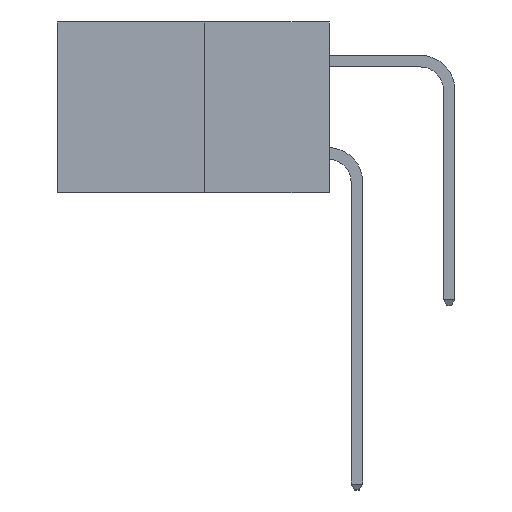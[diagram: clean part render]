
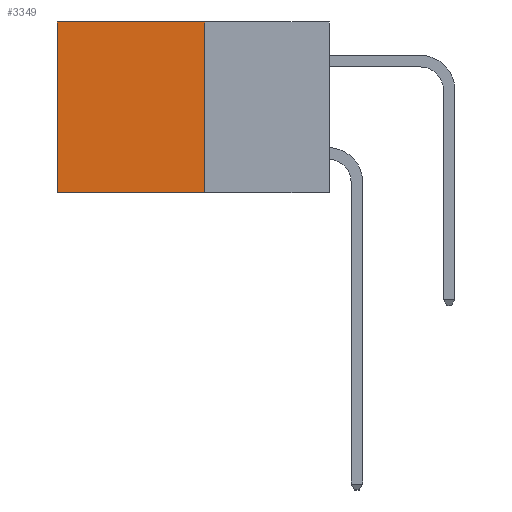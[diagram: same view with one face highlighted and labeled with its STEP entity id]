
A CAD part, left-side view. The second image highlights one B-rep face of the part: STEP entity #3349.
In plain terms, the highlighted planar face has unit normal (-1, 0, 0).
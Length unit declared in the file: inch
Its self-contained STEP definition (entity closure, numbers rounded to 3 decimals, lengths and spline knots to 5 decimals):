
#396 = LINE ( 'NONE', #4796, #4317 ) ;
#1114 = ORIENTED_EDGE ( 'NONE', *, *, #7311, .F. ) ;
#1299 = CARTESIAN_POINT ( 'NONE',  ( 0.277, 0.27, -0.37 ) ) ;
#1785 = LINE ( 'NONE', #10748, #14183 ) ;
#3349 = ADVANCED_FACE ( 'NONE', ( #7899 ), #6500, .F. ) ;
#3978 = DIRECTION ( 'NONE',  ( 0., 0., -1. ) ) ;
#4066 = ORIENTED_EDGE ( 'NONE', *, *, #15987, .F. ) ;
#4118 = AXIS2_PLACEMENT_3D ( 'NONE', #1299, #9331, #3978 ) ;
#4317 = VECTOR ( 'NONE', #13659, 39.37008 ) ;
#4387 = ORIENTED_EDGE ( 'NONE', *, *, #11610, .T. ) ;
#4666 = CARTESIAN_POINT ( 'NONE',  ( 0.277, 0.27, -0.37 ) ) ;
#4796 = CARTESIAN_POINT ( 'NONE',  ( 0.277, 0.27, 0. ) ) ;
#4923 = CARTESIAN_POINT ( 'NONE',  ( 0.277, 0.59, 0. ) ) ;
#5635 = EDGE_LOOP ( 'NONE', ( #4387, #4066, #1114, #10881 ) ) ;
#6076 = VERTEX_POINT ( 'NONE', #4923 ) ;
#6500 = PLANE ( 'NONE',  #4118 ) ;
#6636 = EDGE_CURVE ( 'NONE', #11282, #6076, #396, .T. ) ;
#7311 = EDGE_CURVE ( 'NONE', #11282, #11649, #13811, .T. ) ;
#7348 = LINE ( 'NONE', #8832, #13654 ) ;
#7899 = FACE_OUTER_BOUND ( 'NONE', #5635, .T. ) ;
#8777 = CARTESIAN_POINT ( 'NONE',  ( 0.277, 0.59, -0.37 ) ) ;
#8832 = CARTESIAN_POINT ( 'NONE',  ( 0.277, 0.27, -0.37 ) ) ;
#9331 = DIRECTION ( 'NONE',  ( 1., 0., 0. ) ) ;
#10033 = CARTESIAN_POINT ( 'NONE',  ( 0.277, 0.27, 0. ) ) ;
#10103 = DIRECTION ( 'NONE',  ( 0., 1., 0. ) ) ;
#10471 = VECTOR ( 'NONE', #12311, 39.37008 ) ;
#10748 = CARTESIAN_POINT ( 'NONE',  ( 0.277, 0.59, -0.37 ) ) ;
#10881 = ORIENTED_EDGE ( 'NONE', *, *, #6636, .T. ) ;
#11282 = VERTEX_POINT ( 'NONE', #10033 ) ;
#11610 = EDGE_CURVE ( 'NONE', #6076, #15957, #1785, .T. ) ;
#11649 = VERTEX_POINT ( 'NONE', #14563 ) ;
#12002 = DIRECTION ( 'NONE',  ( 0., 0., -1. ) ) ;
#12311 = DIRECTION ( 'NONE',  ( 0., 0., -1. ) ) ;
#13654 = VECTOR ( 'NONE', #10103, 39.37008 ) ;
#13659 = DIRECTION ( 'NONE',  ( 0., 1., 0. ) ) ;
#13811 = LINE ( 'NONE', #4666, #10471 ) ;
#14183 = VECTOR ( 'NONE', #12002, 39.37008 ) ;
#14563 = CARTESIAN_POINT ( 'NONE',  ( 0.277, 0.27, -0.37 ) ) ;
#15957 = VERTEX_POINT ( 'NONE', #8777 ) ;
#15987 = EDGE_CURVE ( 'NONE', #11649, #15957, #7348, .T. ) ;
